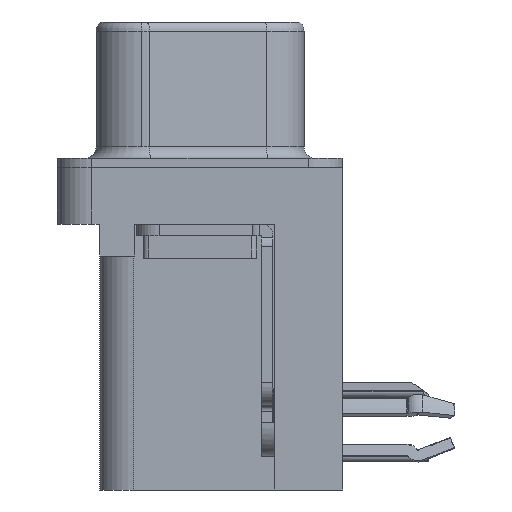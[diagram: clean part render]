
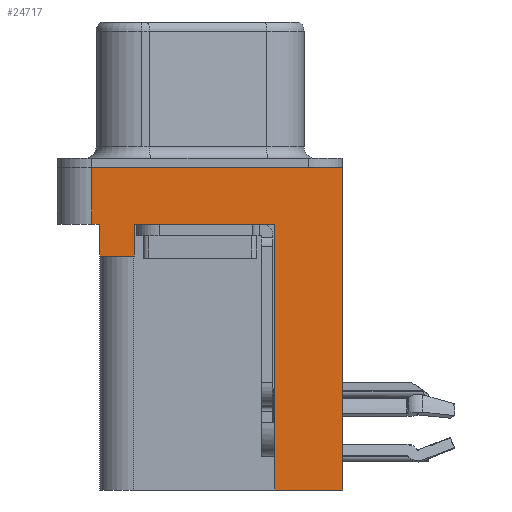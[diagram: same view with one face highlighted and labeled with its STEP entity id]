
A CAD part, left-side view. The second image highlights one B-rep face of the part: STEP entity #24717.
In plain terms, the highlighted planar face has unit normal (-1, 0, 0).
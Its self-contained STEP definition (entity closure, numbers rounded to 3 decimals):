
#462 = CARTESIAN_POINT ( 'NONE',  ( -2.91, 4.775, 0. ) ) ;
#620 = CARTESIAN_POINT ( 'NONE',  ( -2.91, -6.275, 0. ) ) ;
#967 = VECTOR ( 'NONE', #7509, 1000. ) ;
#1019 = DIRECTION ( 'NONE',  ( -1., 0., 0. ) ) ;
#1351 = ORIENTED_EDGE ( 'NONE', *, *, #6620, .T. ) ;
#1466 = DIRECTION ( 'NONE',  ( 0., -1., 0. ) ) ;
#1553 = VERTEX_POINT ( 'NONE', #8806 ) ;
#2193 = VERTEX_POINT ( 'NONE', #620 ) ;
#2483 = CARTESIAN_POINT ( 'NONE',  ( -2.91, -6.275, -14.2 ) ) ;
#3208 = CARTESIAN_POINT ( 'NONE',  ( -2.91, -6.275, 0. ) ) ;
#4055 = CARTESIAN_POINT ( 'NONE',  ( -2.91, -6.275, -2.5 ) ) ;
#4324 = EDGE_CURVE ( 'NONE', #28026, #2193, #13922, .T. ) ;
#4548 = VECTOR ( 'NONE', #21516, 1000. ) ;
#6175 = ORIENTED_EDGE ( 'NONE', *, *, #28142, .F. ) ;
#6571 = ORIENTED_EDGE ( 'NONE', *, *, #12840, .F. ) ;
#6620 = EDGE_CURVE ( 'NONE', #24948, #1553, #11938, .T. ) ;
#6834 = CARTESIAN_POINT ( 'NONE',  ( -2.91, 4.775, -2.5 ) ) ;
#7197 = DIRECTION ( 'NONE',  ( 0., 0., 1. ) ) ;
#7203 = DIRECTION ( 'NONE',  ( 0., 0., 1. ) ) ;
#7334 = FACE_OUTER_BOUND ( 'NONE', #11305, .T. ) ;
#7352 = VERTEX_POINT ( 'NONE', #17176 ) ;
#7468 = DIRECTION ( 'NONE',  ( 0., 0., 1. ) ) ;
#7509 = DIRECTION ( 'NONE',  ( 0., 0., 1. ) ) ;
#8326 = VERTEX_POINT ( 'NONE', #16346 ) ;
#8382 = VECTOR ( 'NONE', #7203, 1000. ) ;
#8472 = CARTESIAN_POINT ( 'NONE',  ( -2.91, 4.425, -3.9 ) ) ;
#8806 = CARTESIAN_POINT ( 'NONE',  ( -2.91, 2.895, -2.5 ) ) ;
#8848 = EDGE_CURVE ( 'NONE', #22578, #2193, #14155, .T. ) ;
#8989 = DIRECTION ( 'NONE',  ( 0., 1., 0. ) ) ;
#9280 = LINE ( 'NONE', #26717, #24666 ) ;
#9603 = PLANE ( 'NONE',  #26721 ) ;
#10444 = CARTESIAN_POINT ( 'NONE',  ( -2.91, 4.775, -2.5 ) ) ;
#10523 = EDGE_CURVE ( 'NONE', #22578, #7352, #9280, .T. ) ;
#11007 = ORIENTED_EDGE ( 'NONE', *, *, #23174, .F. ) ;
#11184 = ORIENTED_EDGE ( 'NONE', *, *, #8848, .T. ) ;
#11305 = EDGE_LOOP ( 'NONE', ( #25680, #6571, #24375, #6175, #11007, #1351, #21256, #11753, #26712, #11184 ) ) ;
#11753 = ORIENTED_EDGE ( 'NONE', *, *, #26197, .F. ) ;
#11922 = DIRECTION ( 'NONE',  ( 0., -1., 0. ) ) ;
#11938 = LINE ( 'NONE', #22794, #22764 ) ;
#12840 = EDGE_CURVE ( 'NONE', #16960, #28026, #14192, .T. ) ;
#12880 = LINE ( 'NONE', #8472, #24876 ) ;
#13922 = LINE ( 'NONE', #3208, #21330 ) ;
#14155 = LINE ( 'NONE', #22598, #20611 ) ;
#14192 = LINE ( 'NONE', #10444, #967 ) ;
#14472 = LINE ( 'NONE', #4055, #26940 ) ;
#15520 = EDGE_CURVE ( 'NONE', #16960, #22630, #24958, .T. ) ;
#16104 = EDGE_CURVE ( 'NONE', #1553, #8326, #14472, .T. ) ;
#16316 = CARTESIAN_POINT ( 'NONE',  ( -2.91, -3.295, -14.2 ) ) ;
#16346 = CARTESIAN_POINT ( 'NONE',  ( -2.91, -3.295, -2.5 ) ) ;
#16374 = DIRECTION ( 'NONE',  ( 0., 0., 1. ) ) ;
#16558 = CARTESIAN_POINT ( 'NONE',  ( -2.91, 4.425, -3.9 ) ) ;
#16960 = VERTEX_POINT ( 'NONE', #6834 ) ;
#17176 = CARTESIAN_POINT ( 'NONE',  ( -2.91, -3.295, -14.2 ) ) ;
#17181 = DIRECTION ( 'NONE',  ( 0., 1., 0. ) ) ;
#17893 = CARTESIAN_POINT ( 'NONE',  ( -2.91, -6.275, -2.5 ) ) ;
#20611 = VECTOR ( 'NONE', #7197, 1000. ) ;
#21133 = DIRECTION ( 'NONE',  ( 0., 0., 1. ) ) ;
#21158 = CARTESIAN_POINT ( 'NONE',  ( -2.91, 2.895, -3.9 ) ) ;
#21256 = ORIENTED_EDGE ( 'NONE', *, *, #16104, .T. ) ;
#21330 = VECTOR ( 'NONE', #11922, 1000. ) ;
#21516 = DIRECTION ( 'NONE',  ( 0., -1., 0. ) ) ;
#22354 = CARTESIAN_POINT ( 'NONE',  ( -2.91, 4.425, -2.5 ) ) ;
#22578 = VERTEX_POINT ( 'NONE', #2483 ) ;
#22598 = CARTESIAN_POINT ( 'NONE',  ( -2.91, -6.275, -2.5 ) ) ;
#22630 = VERTEX_POINT ( 'NONE', #22354 ) ;
#22717 = VERTEX_POINT ( 'NONE', #26364 ) ;
#22764 = VECTOR ( 'NONE', #16374, 1000. ) ;
#22794 = CARTESIAN_POINT ( 'NONE',  ( -2.91, 2.895, -3.9 ) ) ;
#22883 = LINE ( 'NONE', #16316, #8382 ) ;
#23174 = EDGE_CURVE ( 'NONE', #24948, #22717, #12880, .T. ) ;
#24375 = ORIENTED_EDGE ( 'NONE', *, *, #15520, .T. ) ;
#24666 = VECTOR ( 'NONE', #8989, 1000. ) ;
#24717 = ADVANCED_FACE ( 'NONE', ( #7334 ), #9603, .T. ) ;
#24876 = VECTOR ( 'NONE', #17181, 1000. ) ;
#24948 = VERTEX_POINT ( 'NONE', #21158 ) ;
#24958 = LINE ( 'NONE', #26085, #4548 ) ;
#25680 = ORIENTED_EDGE ( 'NONE', *, *, #4324, .F. ) ;
#26085 = CARTESIAN_POINT ( 'NONE',  ( -2.91, -6.275, -2.5 ) ) ;
#26197 = EDGE_CURVE ( 'NONE', #7352, #8326, #22883, .T. ) ;
#26364 = CARTESIAN_POINT ( 'NONE',  ( -2.91, 4.425, -3.9 ) ) ;
#26665 = VECTOR ( 'NONE', #21133, 1000. ) ;
#26712 = ORIENTED_EDGE ( 'NONE', *, *, #10523, .F. ) ;
#26717 = CARTESIAN_POINT ( 'NONE',  ( -2.91, -3.295, -14.2 ) ) ;
#26721 = AXIS2_PLACEMENT_3D ( 'NONE', #17893, #1019, #7468 ) ;
#26940 = VECTOR ( 'NONE', #1466, 1000. ) ;
#27851 = LINE ( 'NONE', #16558, #26665 ) ;
#28026 = VERTEX_POINT ( 'NONE', #462 ) ;
#28142 = EDGE_CURVE ( 'NONE', #22717, #22630, #27851, .T. ) ;
